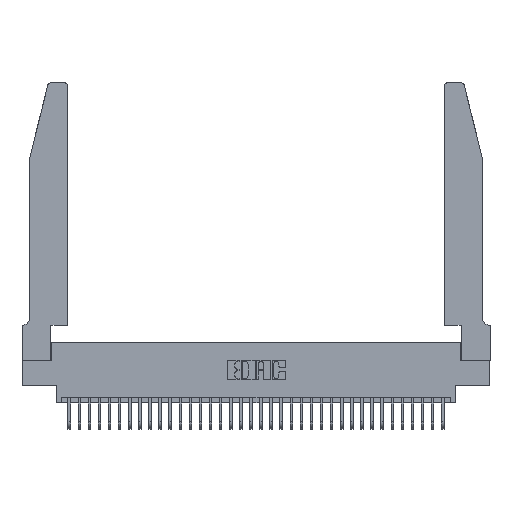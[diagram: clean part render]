
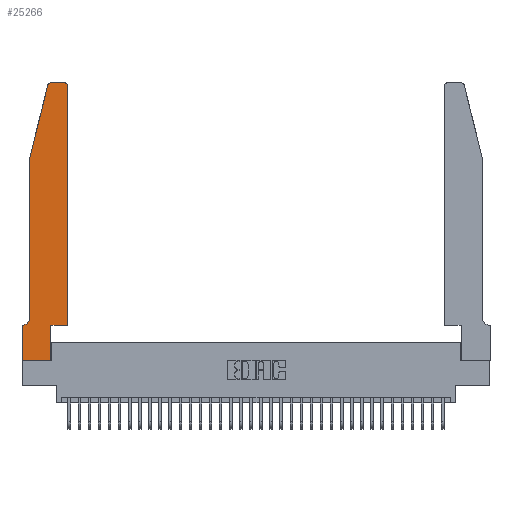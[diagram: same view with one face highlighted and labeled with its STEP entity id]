
A CAD part, top view. The second image highlights one B-rep face of the part: STEP entity #25266.
In plain terms, the highlighted planar face has unit normal (0, 0, 1).
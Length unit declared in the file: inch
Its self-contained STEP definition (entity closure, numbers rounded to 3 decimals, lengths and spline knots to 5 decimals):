
#1050 = VECTOR ( 'NONE', #21925, 39.37008 ) ;
#1074 = DIRECTION ( 'NONE',  ( 0., 0., 1. ) ) ;
#1296 = CARTESIAN_POINT ( 'NONE',  ( 0.0755, 2., 0.37 ) ) ;
#1359 = VERTEX_POINT ( 'NONE', #11884 ) ;
#2157 = ORIENTED_EDGE ( 'NONE', *, *, #8704, .T. ) ;
#2403 = DIRECTION ( 'NONE',  ( 0., 0., -1. ) ) ;
#3518 = LINE ( 'NONE', #25132, #34299 ) ;
#3970 = VECTOR ( 'NONE', #12788, 39.37008 ) ;
#4140 = EDGE_CURVE ( 'NONE', #8004, #16013, #13292, .T. ) ;
#4256 = CARTESIAN_POINT ( 'NONE',  ( 0.284, 2.72, 0.37 ) ) ;
#4697 = CARTESIAN_POINT ( 'NONE',  ( 0.0755, 0.35, 0.37 ) ) ;
#5046 = DIRECTION ( 'NONE',  ( 1., 0., 0. ) ) ;
#5945 = CARTESIAN_POINT ( 'NONE',  ( 0., 0.35, 0.37 ) ) ;
#6331 = CARTESIAN_POINT ( 'NONE',  ( 0.4505, 2.72, 0.37 ) ) ;
#6335 = ORIENTED_EDGE ( 'NONE', *, *, #31177, .T. ) ;
#6802 = AXIS2_PLACEMENT_3D ( 'NONE', #16426, #22177, #5046 ) ;
#7042 = CARTESIAN_POINT ( 'NONE',  ( 0.4505, 0.35, 0.37 ) ) ;
#7792 = LINE ( 'NONE', #4697, #1050 ) ;
#7912 = ORIENTED_EDGE ( 'NONE', *, *, #18205, .T. ) ;
#8004 = VERTEX_POINT ( 'NONE', #27420 ) ;
#8042 = PLANE ( 'NONE',  #6802 ) ;
#8223 = LINE ( 'NONE', #7042, #13598 ) ;
#8484 = EDGE_CURVE ( 'NONE', #22191, #36427, #36528, .T. ) ;
#8680 = AXIS2_PLACEMENT_3D ( 'NONE', #16641, #2403, #30816 ) ;
#8704 = EDGE_CURVE ( 'NONE', #30561, #11563, #23162, .T. ) ;
#9112 = CARTESIAN_POINT ( 'NONE',  ( 0.0055, 0.35, 0.37 ) ) ;
#10103 = CARTESIAN_POINT ( 'NONE',  ( 0.4505, 0.35, 0.37 ) ) ;
#10321 = EDGE_CURVE ( 'NONE', #29894, #8004, #26732, .T. ) ;
#11139 = DIRECTION ( 'NONE',  ( -1., 0., 0. ) ) ;
#11278 = VECTOR ( 'NONE', #21705, 39.37008 ) ;
#11563 = VERTEX_POINT ( 'NONE', #16931 ) ;
#11884 = CARTESIAN_POINT ( 'NONE',  ( 0.2865, 0.35, 0.37 ) ) ;
#12332 = ORIENTED_EDGE ( 'NONE', *, *, #35192, .T. ) ;
#12613 = ORIENTED_EDGE ( 'NONE', *, *, #16792, .T. ) ;
#12788 = DIRECTION ( 'NONE',  ( 0., -1., 0. ) ) ;
#12845 = CARTESIAN_POINT ( 'NONE',  ( 0.4205, 2.72, 0.37 ) ) ;
#13292 = LINE ( 'NONE', #29910, #27531 ) ;
#13517 = ORIENTED_EDGE ( 'NONE', *, *, #15368, .T. ) ;
#13598 = VECTOR ( 'NONE', #23872, 39.37008 ) ;
#13680 = EDGE_CURVE ( 'NONE', #33699, #29894, #7792, .T. ) ;
#14009 = VECTOR ( 'NONE', #35681, 39.37008 ) ;
#14296 = VERTEX_POINT ( 'NONE', #10103 ) ;
#15036 = ORIENTED_EDGE ( 'NONE', *, *, #10321, .T. ) ;
#15345 = ORIENTED_EDGE ( 'NONE', *, *, #22321, .T. ) ;
#15368 = EDGE_CURVE ( 'NONE', #1359, #14296, #8223, .T. ) ;
#15593 = VECTOR ( 'NONE', #30596, 39.37008 ) ;
#16013 = VERTEX_POINT ( 'NONE', #30366 ) ;
#16157 = VECTOR ( 'NONE', #11139, 39.37008 ) ;
#16316 = CARTESIAN_POINT ( 'NONE',  ( 0.0755, 0.42, 0.37 ) ) ;
#16426 = CARTESIAN_POINT ( 'NONE',  ( 0., 0.35, 0.37 ) ) ;
#16641 = CARTESIAN_POINT ( 'NONE',  ( 0.0055, 0.42, 0.37 ) ) ;
#16792 = EDGE_CURVE ( 'NONE', #11563, #30409, #21539, .T. ) ;
#16931 = CARTESIAN_POINT ( 'NONE',  ( 0.0755, 2., 0.37 ) ) ;
#16954 = DIRECTION ( 'NONE',  ( 0., 1., 0. ) ) ;
#17040 = CARTESIAN_POINT ( 'NONE',  ( 0.25487, 2.72718, 0.37 ) ) ;
#17519 = CIRCLE ( 'NONE', #8680, 0.07 ) ;
#18205 = EDGE_CURVE ( 'NONE', #16013, #1359, #3518, .T. ) ;
#18231 = CARTESIAN_POINT ( 'NONE',  ( 0., 0., 0.37 ) ) ;
#19265 = LINE ( 'NONE', #36530, #16157 ) ;
#19605 = ORIENTED_EDGE ( 'NONE', *, *, #8484, .T. ) ;
#19765 = LINE ( 'NONE', #32888, #11278 ) ;
#20029 = VERTEX_POINT ( 'NONE', #32857 ) ;
#21535 = AXIS2_PLACEMENT_3D ( 'NONE', #12845, #1074, #32613 ) ;
#21539 = LINE ( 'NONE', #24494, #14009 ) ;
#21705 = DIRECTION ( 'NONE',  ( 0., 1., 0. ) ) ;
#21925 = DIRECTION ( 'NONE',  ( -1., 0., 0. ) ) ;
#22177 = DIRECTION ( 'NONE',  ( 0., 0., 1. ) ) ;
#22191 = VERTEX_POINT ( 'NONE', #6331 ) ;
#22321 = EDGE_CURVE ( 'NONE', #14296, #22191, #19765, .T. ) ;
#23066 = EDGE_CURVE ( 'NONE', #36427, #20029, #19265, .T. ) ;
#23162 = LINE ( 'NONE', #1296, #15593 ) ;
#23872 = DIRECTION ( 'NONE',  ( 1., 0., 0. ) ) ;
#24494 = CARTESIAN_POINT ( 'NONE',  ( 0.0755, 2., 0.37 ) ) ;
#25132 = CARTESIAN_POINT ( 'NONE',  ( 0.2865, 0.35, 0.37 ) ) ;
#25266 = ADVANCED_FACE ( 'NONE', ( #30717 ), #8042, .T. ) ;
#26732 = LINE ( 'NONE', #18231, #3970 ) ;
#26823 = DIRECTION ( 'NONE',  ( 0., 0., 1. ) ) ;
#27035 = CIRCLE ( 'NONE', #27611, 0.03 ) ;
#27216 = DIRECTION ( 'NONE',  ( 1., 0., 0. ) ) ;
#27420 = CARTESIAN_POINT ( 'NONE',  ( 0., 0., 0.37 ) ) ;
#27531 = VECTOR ( 'NONE', #27216, 39.37008 ) ;
#27611 = AXIS2_PLACEMENT_3D ( 'NONE', #4256, #26823, #32541 ) ;
#29894 = VERTEX_POINT ( 'NONE', #5945 ) ;
#29910 = CARTESIAN_POINT ( 'NONE',  ( 0., 0., 0.37 ) ) ;
#30366 = CARTESIAN_POINT ( 'NONE',  ( 0.2865, 0., 0.37 ) ) ;
#30409 = VERTEX_POINT ( 'NONE', #16316 ) ;
#30561 = VERTEX_POINT ( 'NONE', #17040 ) ;
#30596 = DIRECTION ( 'NONE',  ( -0.239, -0.971, 0. ) ) ;
#30717 = FACE_OUTER_BOUND ( 'NONE', #32331, .T. ) ;
#30816 = DIRECTION ( 'NONE',  ( -1., 0., 0. ) ) ;
#31177 = EDGE_CURVE ( 'NONE', #30409, #33699, #17519, .T. ) ;
#32013 = ORIENTED_EDGE ( 'NONE', *, *, #13680, .T. ) ;
#32331 = EDGE_LOOP ( 'NONE', ( #34124, #12332, #2157, #12613, #6335, #32013, #15036, #33303, #7912, #13517, #15345, #19605 ) ) ;
#32541 = DIRECTION ( 'NONE',  ( 1., 0., 0. ) ) ;
#32613 = DIRECTION ( 'NONE',  ( 1., 0., 0. ) ) ;
#32857 = CARTESIAN_POINT ( 'NONE',  ( 0.284, 2.75, 0.37 ) ) ;
#32888 = CARTESIAN_POINT ( 'NONE',  ( 0.4505, 0.35, 0.37 ) ) ;
#33303 = ORIENTED_EDGE ( 'NONE', *, *, #4140, .T. ) ;
#33699 = VERTEX_POINT ( 'NONE', #9112 ) ;
#34124 = ORIENTED_EDGE ( 'NONE', *, *, #23066, .T. ) ;
#34299 = VECTOR ( 'NONE', #16954, 39.37008 ) ;
#34816 = CARTESIAN_POINT ( 'NONE',  ( 0.4205, 2.75, 0.37 ) ) ;
#35192 = EDGE_CURVE ( 'NONE', #20029, #30561, #27035, .T. ) ;
#35681 = DIRECTION ( 'NONE',  ( 0., -1., 0. ) ) ;
#36427 = VERTEX_POINT ( 'NONE', #34816 ) ;
#36528 = CIRCLE ( 'NONE', #21535, 0.03 ) ;
#36530 = CARTESIAN_POINT ( 'NONE',  ( 0.2605, 2.75, 0.37 ) ) ;
